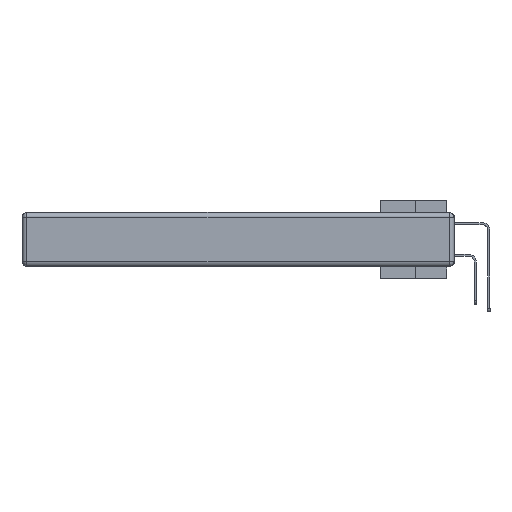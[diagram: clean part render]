
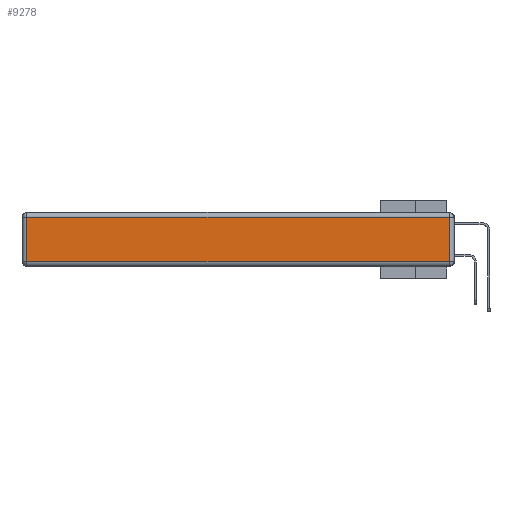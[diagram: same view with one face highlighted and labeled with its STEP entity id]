
A CAD part, left-side view. The second image highlights one B-rep face of the part: STEP entity #9278.
In plain terms, the highlighted planar face has unit normal (-1, 0, 0).
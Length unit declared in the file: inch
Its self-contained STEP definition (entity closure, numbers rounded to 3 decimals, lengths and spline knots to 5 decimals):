
#2100 = EDGE_CURVE ( 'NONE', #37411, #2789, #6886, .T. ) ;
#2789 = VERTEX_POINT ( 'NONE', #8746 ) ;
#2928 = ORIENTED_EDGE ( 'NONE', *, *, #19143, .T. ) ;
#3414 = VECTOR ( 'NONE', #9810, 39.37008 ) ;
#3491 = VECTOR ( 'NONE', #27411, 39.37008 ) ;
#6886 = LINE ( 'NONE', #33803, #3414 ) ;
#7719 = CARTESIAN_POINT ( 'NONE',  ( 0., 0., -0.343 ) ) ;
#8746 = CARTESIAN_POINT ( 'NONE',  ( 0., 2.72, -0.03 ) ) ;
#9278 = ADVANCED_FACE ( 'NONE', ( #10637 ), #22528, .T. ) ;
#9279 = LINE ( 'NONE', #21169, #3491 ) ;
#9810 = DIRECTION ( 'NONE',  ( 0., 1., 0. ) ) ;
#10506 = VERTEX_POINT ( 'NONE', #23446 ) ;
#10637 = FACE_OUTER_BOUND ( 'NONE', #19283, .T. ) ;
#12146 = LINE ( 'NONE', #23847, #12311 ) ;
#12311 = VECTOR ( 'NONE', #30093, 39.37008 ) ;
#14914 = EDGE_CURVE ( 'NONE', #2789, #21872, #35665, .T. ) ;
#19143 = EDGE_CURVE ( 'NONE', #10506, #37411, #12146, .T. ) ;
#19283 = EDGE_LOOP ( 'NONE', ( #27427, #2928, #26739, #33910 ) ) ;
#19601 = DIRECTION ( 'NONE',  ( -1., 0., 0. ) ) ;
#21169 = CARTESIAN_POINT ( 'NONE',  ( 0., 0., -0.313 ) ) ;
#21872 = VERTEX_POINT ( 'NONE', #29954 ) ;
#22528 = PLANE ( 'NONE',  #28793 ) ;
#23446 = CARTESIAN_POINT ( 'NONE',  ( 0., 0.03, -0.313 ) ) ;
#23847 = CARTESIAN_POINT ( 'NONE',  ( 0., 0.03, -0.343 ) ) ;
#23957 = DIRECTION ( 'NONE',  ( 0., 0., -1. ) ) ;
#26315 = CARTESIAN_POINT ( 'NONE',  ( 0., 2.72, -0.343 ) ) ;
#26739 = ORIENTED_EDGE ( 'NONE', *, *, #2100, .T. ) ;
#27411 = DIRECTION ( 'NONE',  ( 0., -1., 0. ) ) ;
#27427 = ORIENTED_EDGE ( 'NONE', *, *, #35326, .T. ) ;
#28573 = DIRECTION ( 'NONE',  ( 0., 0., 1. ) ) ;
#28793 = AXIS2_PLACEMENT_3D ( 'NONE', #7719, #19601, #28573 ) ;
#29091 = CARTESIAN_POINT ( 'NONE',  ( 0., 0.03, -0.03 ) ) ;
#29599 = VECTOR ( 'NONE', #23957, 39.37008 ) ;
#29954 = CARTESIAN_POINT ( 'NONE',  ( 0., 2.72, -0.313 ) ) ;
#30093 = DIRECTION ( 'NONE',  ( 0., 0., 1. ) ) ;
#33803 = CARTESIAN_POINT ( 'NONE',  ( 0., 2.75, -0.03 ) ) ;
#33910 = ORIENTED_EDGE ( 'NONE', *, *, #14914, .T. ) ;
#35326 = EDGE_CURVE ( 'NONE', #21872, #10506, #9279, .T. ) ;
#35665 = LINE ( 'NONE', #26315, #29599 ) ;
#37411 = VERTEX_POINT ( 'NONE', #29091 ) ;
